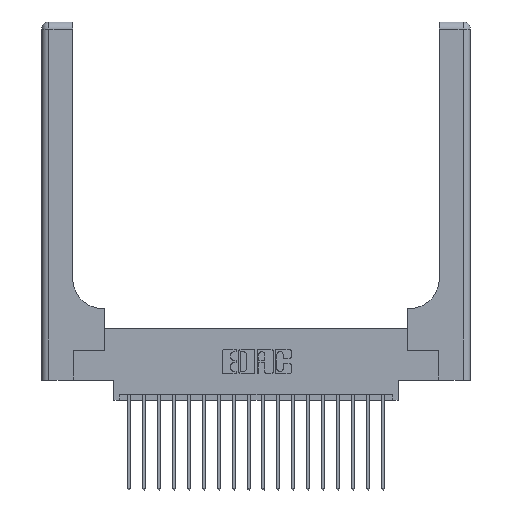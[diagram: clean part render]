
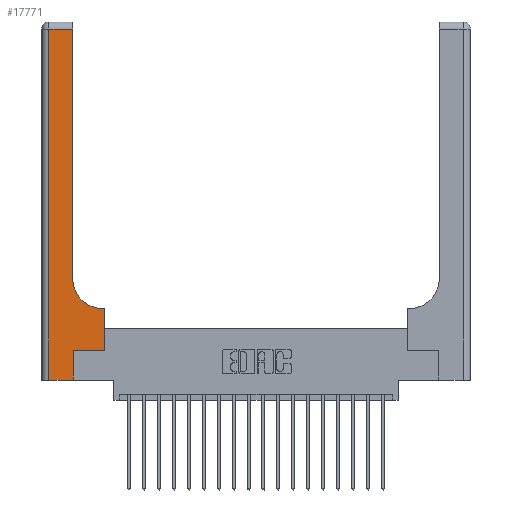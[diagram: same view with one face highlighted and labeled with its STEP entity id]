
A CAD part, top view. The second image highlights one B-rep face of the part: STEP entity #17771.
In plain terms, the highlighted planar face has unit normal (0, 0, 1).
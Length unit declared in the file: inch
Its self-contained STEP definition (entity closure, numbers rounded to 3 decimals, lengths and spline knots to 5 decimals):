
#50 = VERTEX_POINT ( 'NONE', #7658 ) ;
#497 = CARTESIAN_POINT ( 'NONE',  ( 0., 0., 0.37 ) ) ;
#598 = VECTOR ( 'NONE', #4506, 39.37008 ) ;
#707 = LINE ( 'NONE', #6890, #14479 ) ;
#733 = CARTESIAN_POINT ( 'NONE',  ( 0.06, 0., 0.37 ) ) ;
#737 = CARTESIAN_POINT ( 'NONE',  ( 0., 2.94, 0.37 ) ) ;
#1339 = CARTESIAN_POINT ( 'NONE',  ( 0.265, 0.25, 0.37 ) ) ;
#1484 = FACE_OUTER_BOUND ( 'NONE', #16396, .T. ) ;
#1654 = ORIENTED_EDGE ( 'NONE', *, *, #20000, .T. ) ;
#2419 = VECTOR ( 'NONE', #18508, 39.37008 ) ;
#2459 = DIRECTION ( 'NONE',  ( 0., -1., 0. ) ) ;
#2986 = AXIS2_PLACEMENT_3D ( 'NONE', #14640, #9744, #17956 ) ;
#3040 = EDGE_CURVE ( 'NONE', #20646, #50, #15848, .T. ) ;
#3237 = LINE ( 'NONE', #20469, #14569 ) ;
#3882 = DIRECTION ( 'NONE',  ( 0., 1., 0. ) ) ;
#4506 = DIRECTION ( 'NONE',  ( 1., 0., 0. ) ) ;
#4546 = ORIENTED_EDGE ( 'NONE', *, *, #16170, .T. ) ;
#4572 = LINE ( 'NONE', #10998, #7496 ) ;
#5478 = VERTEX_POINT ( 'NONE', #8554 ) ;
#5961 = DIRECTION ( 'NONE',  ( 0., 1., 0. ) ) ;
#6096 = EDGE_CURVE ( 'NONE', #50, #15755, #9145, .T. ) ;
#6108 = VERTEX_POINT ( 'NONE', #13740 ) ;
#6191 = ORIENTED_EDGE ( 'NONE', *, *, #11265, .T. ) ;
#6202 = DIRECTION ( 'NONE',  ( 0., 1., 0. ) ) ;
#6890 = CARTESIAN_POINT ( 'NONE',  ( 0.26, 3., 0.37 ) ) ;
#7496 = VECTOR ( 'NONE', #2459, 39.37008 ) ;
#7545 = LINE ( 'NONE', #737, #14183 ) ;
#7658 = CARTESIAN_POINT ( 'NONE',  ( 0.528, 0.25, 0.37 ) ) ;
#8521 = VERTEX_POINT ( 'NONE', #18395 ) ;
#8554 = CARTESIAN_POINT ( 'NONE',  ( 0.265, 0., 0.37 ) ) ;
#9145 = LINE ( 'NONE', #12197, #18475 ) ;
#9216 = ORIENTED_EDGE ( 'NONE', *, *, #12761, .T. ) ;
#9526 = ORIENTED_EDGE ( 'NONE', *, *, #11030, .T. ) ;
#9669 = CARTESIAN_POINT ( 'NONE',  ( 0.265, 0.25, 0.37 ) ) ;
#9744 = DIRECTION ( 'NONE',  ( 0., 0., -1. ) ) ;
#9809 = CARTESIAN_POINT ( 'NONE',  ( 0.26, 2.94, 0.37 ) ) ;
#9907 = LINE ( 'NONE', #16299, #14269 ) ;
#10514 = ORIENTED_EDGE ( 'NONE', *, *, #13663, .T. ) ;
#10998 = CARTESIAN_POINT ( 'NONE',  ( 0.06, 3., 0.37 ) ) ;
#11030 = EDGE_CURVE ( 'NONE', #8521, #12223, #707, .T. ) ;
#11265 = EDGE_CURVE ( 'NONE', #17840, #17471, #4572, .T. ) ;
#11293 = CARTESIAN_POINT ( 'NONE',  ( 0., 3., 0.37 ) ) ;
#11900 = CARTESIAN_POINT ( 'NONE',  ( 0.06, 2.94, 0.37 ) ) ;
#12197 = CARTESIAN_POINT ( 'NONE',  ( 0.528, 0.25, 0.37 ) ) ;
#12223 = VERTEX_POINT ( 'NONE', #9809 ) ;
#12388 = ORIENTED_EDGE ( 'NONE', *, *, #15354, .T. ) ;
#12761 = EDGE_CURVE ( 'NONE', #5478, #20646, #3237, .T. ) ;
#13443 = LINE ( 'NONE', #497, #2419 ) ;
#13663 = EDGE_CURVE ( 'NONE', #15755, #6108, #9907, .T. ) ;
#13740 = CARTESIAN_POINT ( 'NONE',  ( 0.51, 0.6, 0.37 ) ) ;
#14183 = VECTOR ( 'NONE', #18619, 39.37008 ) ;
#14269 = VECTOR ( 'NONE', #19768, 39.37008 ) ;
#14299 = PLANE ( 'NONE',  #17584 ) ;
#14479 = VECTOR ( 'NONE', #3882, 39.37008 ) ;
#14569 = VECTOR ( 'NONE', #6202, 39.37008 ) ;
#14640 = CARTESIAN_POINT ( 'NONE',  ( 0.51, 0.85, 0.37 ) ) ;
#15354 = EDGE_CURVE ( 'NONE', #12223, #17840, #7545, .T. ) ;
#15392 = CIRCLE ( 'NONE', #2986, 0.25 ) ;
#15755 = VERTEX_POINT ( 'NONE', #17000 ) ;
#15848 = LINE ( 'NONE', #1339, #598 ) ;
#16170 = EDGE_CURVE ( 'NONE', #17471, #5478, #13443, .T. ) ;
#16299 = CARTESIAN_POINT ( 'NONE',  ( 0.26, 0.6, 0.37 ) ) ;
#16396 = EDGE_LOOP ( 'NONE', ( #9526, #12388, #6191, #4546, #9216, #20744, #18336, #10514, #1654 ) ) ;
#17000 = CARTESIAN_POINT ( 'NONE',  ( 0.528, 0.6, 0.37 ) ) ;
#17471 = VERTEX_POINT ( 'NONE', #733 ) ;
#17584 = AXIS2_PLACEMENT_3D ( 'NONE', #11293, #19258, #20696 ) ;
#17771 = ADVANCED_FACE ( 'NONE', ( #1484 ), #14299, .F. ) ;
#17840 = VERTEX_POINT ( 'NONE', #11900 ) ;
#17956 = DIRECTION ( 'NONE',  ( 1., 0., 0. ) ) ;
#18336 = ORIENTED_EDGE ( 'NONE', *, *, #6096, .T. ) ;
#18395 = CARTESIAN_POINT ( 'NONE',  ( 0.26, 0.85, 0.37 ) ) ;
#18475 = VECTOR ( 'NONE', #5961, 39.37008 ) ;
#18508 = DIRECTION ( 'NONE',  ( 1., 0., 0. ) ) ;
#18619 = DIRECTION ( 'NONE',  ( -1., 0., 0. ) ) ;
#19258 = DIRECTION ( 'NONE',  ( 0., 0., -1. ) ) ;
#19768 = DIRECTION ( 'NONE',  ( -1., 0., 0. ) ) ;
#20000 = EDGE_CURVE ( 'NONE', #6108, #8521, #15392, .T. ) ;
#20469 = CARTESIAN_POINT ( 'NONE',  ( 0.265, 0., 0.37 ) ) ;
#20646 = VERTEX_POINT ( 'NONE', #9669 ) ;
#20696 = DIRECTION ( 'NONE',  ( -1., 0., 0. ) ) ;
#20744 = ORIENTED_EDGE ( 'NONE', *, *, #3040, .T. ) ;
